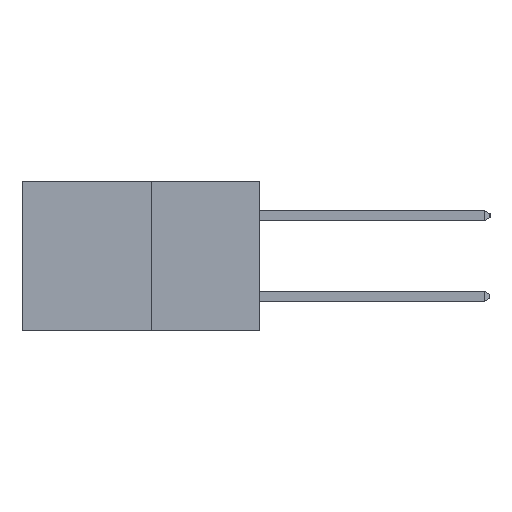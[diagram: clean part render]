
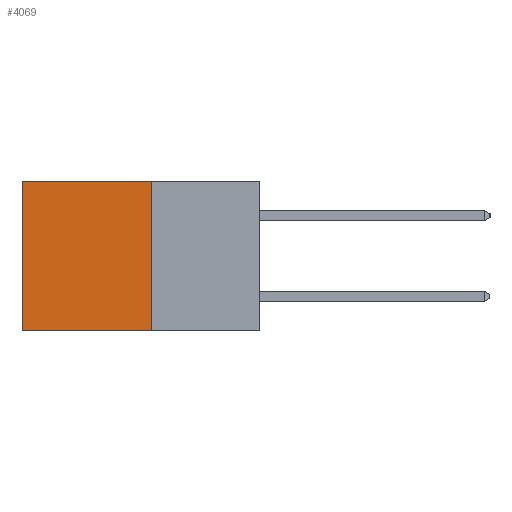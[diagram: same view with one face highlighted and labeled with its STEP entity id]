
A CAD part, left-side view. The second image highlights one B-rep face of the part: STEP entity #4069.
In plain terms, the highlighted planar face has unit normal (-1, 0, 0).
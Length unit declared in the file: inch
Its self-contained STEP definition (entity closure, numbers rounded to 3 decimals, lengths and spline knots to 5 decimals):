
#86 = ORIENTED_EDGE ( 'NONE', *, *, #9255, .F. ) ;
#286 = VERTEX_POINT ( 'NONE', #8383 ) ;
#388 = DIRECTION ( 'NONE',  ( 0., 0., -1. ) ) ;
#498 = CARTESIAN_POINT ( 'NONE',  ( 0.277, 0.59, 0. ) ) ;
#942 = CARTESIAN_POINT ( 'NONE',  ( 0.277, 0.59, -0.37 ) ) ;
#1328 = LINE ( 'NONE', #1713, #10078 ) ;
#1648 = AXIS2_PLACEMENT_3D ( 'NONE', #12044, #12024, #11988 ) ;
#1713 = CARTESIAN_POINT ( 'NONE',  ( 0.277, 0.27, -0.37 ) ) ;
#3889 = EDGE_LOOP ( 'NONE', ( #13652, #14285, #86, #11133 ) ) ;
#4069 = ADVANCED_FACE ( 'NONE', ( #10724 ), #12399, .F. ) ;
#4154 = VECTOR ( 'NONE', #388, 39.37008 ) ;
#4718 = CARTESIAN_POINT ( 'NONE',  ( 0.277, 0.27, 0. ) ) ;
#4932 = VERTEX_POINT ( 'NONE', #498 ) ;
#5229 = LINE ( 'NONE', #9451, #4154 ) ;
#6502 = LINE ( 'NONE', #11127, #9155 ) ;
#7029 = DIRECTION ( 'NONE',  ( 0., 1., 0. ) ) ;
#7354 = VERTEX_POINT ( 'NONE', #942 ) ;
#8241 = EDGE_CURVE ( 'NONE', #11807, #4932, #14035, .T. ) ;
#8383 = CARTESIAN_POINT ( 'NONE',  ( 0.277, 0.27, -0.37 ) ) ;
#8503 = EDGE_CURVE ( 'NONE', #286, #7354, #1328, .T. ) ;
#8797 = DIRECTION ( 'NONE',  ( 0., 0., -1. ) ) ;
#9155 = VECTOR ( 'NONE', #8797, 39.37008 ) ;
#9255 = EDGE_CURVE ( 'NONE', #11807, #286, #6502, .T. ) ;
#9451 = CARTESIAN_POINT ( 'NONE',  ( 0.277, 0.59, -0.37 ) ) ;
#10078 = VECTOR ( 'NONE', #13153, 39.37008 ) ;
#10292 = EDGE_CURVE ( 'NONE', #4932, #7354, #5229, .T. ) ;
#10608 = VECTOR ( 'NONE', #7029, 39.37008 ) ;
#10724 = FACE_OUTER_BOUND ( 'NONE', #3889, .T. ) ;
#11127 = CARTESIAN_POINT ( 'NONE',  ( 0.277, 0.27, -0.37 ) ) ;
#11133 = ORIENTED_EDGE ( 'NONE', *, *, #8241, .T. ) ;
#11807 = VERTEX_POINT ( 'NONE', #13339 ) ;
#11988 = DIRECTION ( 'NONE',  ( 0., 0., -1. ) ) ;
#12024 = DIRECTION ( 'NONE',  ( 1., 0., 0. ) ) ;
#12044 = CARTESIAN_POINT ( 'NONE',  ( 0.277, 0.27, -0.37 ) ) ;
#12399 = PLANE ( 'NONE',  #1648 ) ;
#13153 = DIRECTION ( 'NONE',  ( 0., 1., 0. ) ) ;
#13339 = CARTESIAN_POINT ( 'NONE',  ( 0.277, 0.27, 0. ) ) ;
#13652 = ORIENTED_EDGE ( 'NONE', *, *, #10292, .T. ) ;
#14035 = LINE ( 'NONE', #4718, #10608 ) ;
#14285 = ORIENTED_EDGE ( 'NONE', *, *, #8503, .F. ) ;
